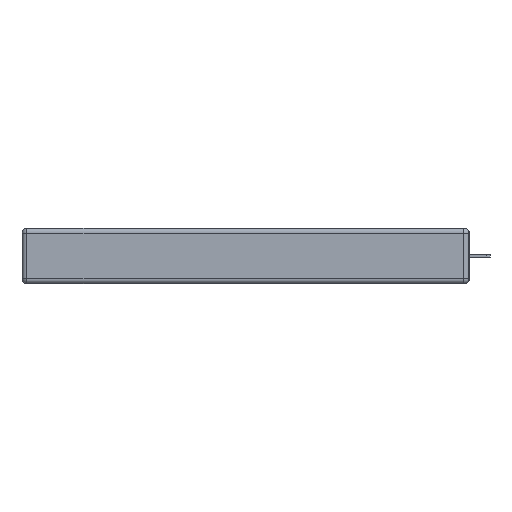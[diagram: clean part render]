
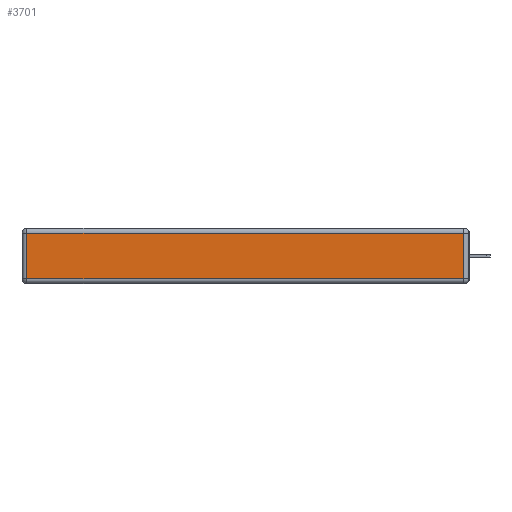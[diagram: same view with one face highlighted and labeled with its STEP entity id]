
A CAD part, left-side view. The second image highlights one B-rep face of the part: STEP entity #3701.
In plain terms, the highlighted planar face has unit normal (-1, 0, 0).
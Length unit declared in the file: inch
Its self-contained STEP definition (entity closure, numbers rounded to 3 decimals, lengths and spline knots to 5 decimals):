
#597 = ORIENTED_EDGE ( 'NONE', *, *, #5601, .T. ) ;
#723 = FACE_OUTER_BOUND ( 'NONE', #14763, .T. ) ;
#927 = DIRECTION ( 'NONE',  ( 0., -1., 0. ) ) ;
#1040 = ORIENTED_EDGE ( 'NONE', *, *, #6494, .T. ) ;
#2207 = CARTESIAN_POINT ( 'NONE',  ( 0., 0.03, -0.343 ) ) ;
#2253 = VECTOR ( 'NONE', #16825, 39.37008 ) ;
#3506 = DIRECTION ( 'NONE',  ( 0., 0., 1. ) ) ;
#3701 = ADVANCED_FACE ( 'NONE', ( #723 ), #6172, .T. ) ;
#3832 = EDGE_CURVE ( 'NONE', #6651, #15162, #12688, .T. ) ;
#3869 = CARTESIAN_POINT ( 'NONE',  ( 0., 0.03, -0.313 ) ) ;
#3969 = CARTESIAN_POINT ( 'NONE',  ( 0., 2.72, -0.03 ) ) ;
#4289 = CARTESIAN_POINT ( 'NONE',  ( 0., 2.75, -0.03 ) ) ;
#4688 = EDGE_CURVE ( 'NONE', #10140, #6651, #5938, .T. ) ;
#5064 = VECTOR ( 'NONE', #3506, 39.37008 ) ;
#5082 = AXIS2_PLACEMENT_3D ( 'NONE', #10064, #15241, #7496 ) ;
#5304 = LINE ( 'NONE', #16597, #8446 ) ;
#5601 = EDGE_CURVE ( 'NONE', #5982, #10140, #12062, .T. ) ;
#5938 = LINE ( 'NONE', #4289, #15873 ) ;
#5982 = VERTEX_POINT ( 'NONE', #3869 ) ;
#6043 = CARTESIAN_POINT ( 'NONE',  ( 0., 0.03, -0.03 ) ) ;
#6172 = PLANE ( 'NONE',  #5082 ) ;
#6494 = EDGE_CURVE ( 'NONE', #15162, #5982, #5304, .T. ) ;
#6651 = VERTEX_POINT ( 'NONE', #3969 ) ;
#7496 = DIRECTION ( 'NONE',  ( 0., 0., 1. ) ) ;
#8151 = CARTESIAN_POINT ( 'NONE',  ( 0., 2.72, -0.313 ) ) ;
#8178 = DIRECTION ( 'NONE',  ( 0., 1., 0. ) ) ;
#8446 = VECTOR ( 'NONE', #927, 39.37008 ) ;
#10064 = CARTESIAN_POINT ( 'NONE',  ( 0., 0., -0.343 ) ) ;
#10140 = VERTEX_POINT ( 'NONE', #6043 ) ;
#10412 = CARTESIAN_POINT ( 'NONE',  ( 0., 2.72, -0.343 ) ) ;
#12062 = LINE ( 'NONE', #2207, #5064 ) ;
#12688 = LINE ( 'NONE', #10412, #2253 ) ;
#14159 = ORIENTED_EDGE ( 'NONE', *, *, #4688, .T. ) ;
#14763 = EDGE_LOOP ( 'NONE', ( #1040, #597, #14159, #15795 ) ) ;
#15162 = VERTEX_POINT ( 'NONE', #8151 ) ;
#15241 = DIRECTION ( 'NONE',  ( -1., 0., 0. ) ) ;
#15795 = ORIENTED_EDGE ( 'NONE', *, *, #3832, .T. ) ;
#15873 = VECTOR ( 'NONE', #8178, 39.37008 ) ;
#16597 = CARTESIAN_POINT ( 'NONE',  ( 0., 0., -0.313 ) ) ;
#16825 = DIRECTION ( 'NONE',  ( 0., 0., -1. ) ) ;
